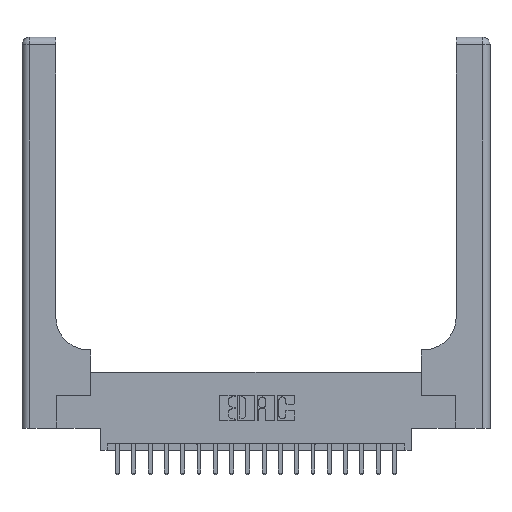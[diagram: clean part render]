
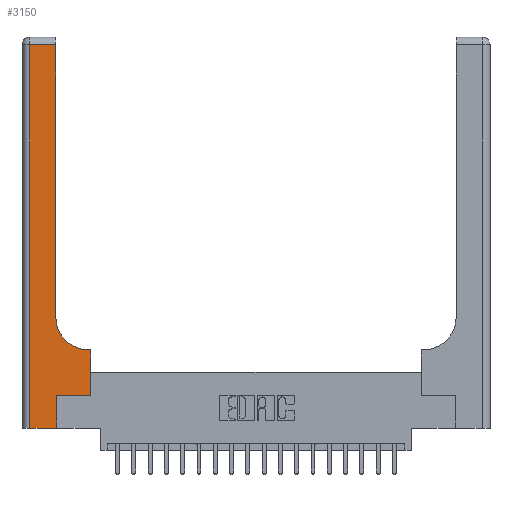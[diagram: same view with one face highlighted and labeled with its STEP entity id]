
A CAD part, top view. The second image highlights one B-rep face of the part: STEP entity #3150.
In plain terms, the highlighted planar face has unit normal (0, 0, 1).
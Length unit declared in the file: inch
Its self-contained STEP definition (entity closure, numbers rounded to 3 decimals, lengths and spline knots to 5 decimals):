
#60 = VERTEX_POINT ( 'NONE', #7449 ) ;
#707 = AXIS2_PLACEMENT_3D ( 'NONE', #6071, #10692, #2780 ) ;
#782 = VECTOR ( 'NONE', #15155, 39.37008 ) ;
#945 = VERTEX_POINT ( 'NONE', #950 ) ;
#950 = CARTESIAN_POINT ( 'NONE',  ( 0.26, 0.85, 0.37 ) ) ;
#1059 = VECTOR ( 'NONE', #18352, 39.37008 ) ;
#1225 = CARTESIAN_POINT ( 'NONE',  ( 0.528, 0.6, 0.37 ) ) ;
#1369 = DIRECTION ( 'NONE',  ( 0., 1., 0. ) ) ;
#1451 = VECTOR ( 'NONE', #9697, 39.37008 ) ;
#2047 = ORIENTED_EDGE ( 'NONE', *, *, #4922, .T. ) ;
#2105 = EDGE_CURVE ( 'NONE', #9536, #15743, #5007, .T. ) ;
#2325 = CARTESIAN_POINT ( 'NONE',  ( 0., 0., 0.37 ) ) ;
#2429 = LINE ( 'NONE', #7509, #1059 ) ;
#2780 = DIRECTION ( 'NONE',  ( -1., 0., 0. ) ) ;
#3150 = ADVANCED_FACE ( 'NONE', ( #20401 ), #20513, .F. ) ;
#3602 = EDGE_CURVE ( 'NONE', #60, #19742, #2429, .T. ) ;
#4331 = LINE ( 'NONE', #10755, #18411 ) ;
#4922 = EDGE_CURVE ( 'NONE', #15743, #9895, #14163, .T. ) ;
#5007 = LINE ( 'NONE', #14596, #5051 ) ;
#5051 = VECTOR ( 'NONE', #13129, 39.37008 ) ;
#5452 = EDGE_CURVE ( 'NONE', #19742, #6913, #15913, .T. ) ;
#5672 = EDGE_CURVE ( 'NONE', #15573, #14285, #19598, .T. ) ;
#5776 = EDGE_CURVE ( 'NONE', #14285, #945, #17637, .T. ) ;
#5795 = EDGE_CURVE ( 'NONE', #945, #9536, #18717, .T. ) ;
#6071 = CARTESIAN_POINT ( 'NONE',  ( 0., 3., 0.37 ) ) ;
#6697 = CARTESIAN_POINT ( 'NONE',  ( 0.06, 0., 0.37 ) ) ;
#6913 = VERTEX_POINT ( 'NONE', #7462 ) ;
#7244 = CARTESIAN_POINT ( 'NONE',  ( 0.26, 3., 0.37 ) ) ;
#7449 = CARTESIAN_POINT ( 'NONE',  ( 0.265, 0., 0.37 ) ) ;
#7462 = CARTESIAN_POINT ( 'NONE',  ( 0.528, 0.25, 0.37 ) ) ;
#7509 = CARTESIAN_POINT ( 'NONE',  ( 0.265, 0., 0.37 ) ) ;
#8540 = AXIS2_PLACEMENT_3D ( 'NONE', #12116, #16936, #18513 ) ;
#8555 = ORIENTED_EDGE ( 'NONE', *, *, #14358, .T. ) ;
#8878 = DIRECTION ( 'NONE',  ( 1., 0., 0. ) ) ;
#9302 = CARTESIAN_POINT ( 'NONE',  ( 0.06, 3., 0.37 ) ) ;
#9536 = VERTEX_POINT ( 'NONE', #17594 ) ;
#9697 = DIRECTION ( 'NONE',  ( 1., 0., 0. ) ) ;
#9891 = VECTOR ( 'NONE', #17103, 39.37008 ) ;
#9895 = VERTEX_POINT ( 'NONE', #6697 ) ;
#10416 = ORIENTED_EDGE ( 'NONE', *, *, #5776, .T. ) ;
#10692 = DIRECTION ( 'NONE',  ( 0., 0., -1. ) ) ;
#10755 = CARTESIAN_POINT ( 'NONE',  ( 0.528, 0.25, 0.37 ) ) ;
#11271 = CARTESIAN_POINT ( 'NONE',  ( 0.265, 0.25, 0.37 ) ) ;
#11497 = ORIENTED_EDGE ( 'NONE', *, *, #3602, .T. ) ;
#12116 = CARTESIAN_POINT ( 'NONE',  ( 0.51, 0.85, 0.37 ) ) ;
#13129 = DIRECTION ( 'NONE',  ( -1., 0., 0. ) ) ;
#13529 = CARTESIAN_POINT ( 'NONE',  ( 0.265, 0.25, 0.37 ) ) ;
#14163 = LINE ( 'NONE', #9302, #9891 ) ;
#14285 = VERTEX_POINT ( 'NONE', #14356 ) ;
#14337 = ORIENTED_EDGE ( 'NONE', *, *, #19873, .T. ) ;
#14356 = CARTESIAN_POINT ( 'NONE',  ( 0.51, 0.6, 0.37 ) ) ;
#14358 = EDGE_CURVE ( 'NONE', #6913, #15573, #4331, .T. ) ;
#14596 = CARTESIAN_POINT ( 'NONE',  ( 0., 2.94, 0.37 ) ) ;
#14755 = ORIENTED_EDGE ( 'NONE', *, *, #5452, .T. ) ;
#15066 = VECTOR ( 'NONE', #8878, 39.37008 ) ;
#15155 = DIRECTION ( 'NONE',  ( -1., 0., 0. ) ) ;
#15512 = ORIENTED_EDGE ( 'NONE', *, *, #5795, .T. ) ;
#15573 = VERTEX_POINT ( 'NONE', #1225 ) ;
#15743 = VERTEX_POINT ( 'NONE', #17677 ) ;
#15913 = LINE ( 'NONE', #11271, #1451 ) ;
#15972 = VECTOR ( 'NONE', #20220, 39.37008 ) ;
#16936 = DIRECTION ( 'NONE',  ( 0., 0., -1. ) ) ;
#17103 = DIRECTION ( 'NONE',  ( 0., -1., 0. ) ) ;
#17174 = ORIENTED_EDGE ( 'NONE', *, *, #2105, .T. ) ;
#17594 = CARTESIAN_POINT ( 'NONE',  ( 0.26, 2.94, 0.37 ) ) ;
#17637 = CIRCLE ( 'NONE', #8540, 0.25 ) ;
#17658 = EDGE_LOOP ( 'NONE', ( #15512, #17174, #2047, #14337, #11497, #14755, #8555, #19809, #10416 ) ) ;
#17677 = CARTESIAN_POINT ( 'NONE',  ( 0.06, 2.94, 0.37 ) ) ;
#18100 = CARTESIAN_POINT ( 'NONE',  ( 0.26, 0.6, 0.37 ) ) ;
#18352 = DIRECTION ( 'NONE',  ( 0., 1., 0. ) ) ;
#18411 = VECTOR ( 'NONE', #1369, 39.37008 ) ;
#18513 = DIRECTION ( 'NONE',  ( 1., 0., 0. ) ) ;
#18567 = LINE ( 'NONE', #2325, #15066 ) ;
#18717 = LINE ( 'NONE', #7244, #15972 ) ;
#19598 = LINE ( 'NONE', #18100, #782 ) ;
#19742 = VERTEX_POINT ( 'NONE', #13529 ) ;
#19809 = ORIENTED_EDGE ( 'NONE', *, *, #5672, .T. ) ;
#19873 = EDGE_CURVE ( 'NONE', #9895, #60, #18567, .T. ) ;
#20220 = DIRECTION ( 'NONE',  ( 0., 1., 0. ) ) ;
#20401 = FACE_OUTER_BOUND ( 'NONE', #17658, .T. ) ;
#20513 = PLANE ( 'NONE',  #707 ) ;
